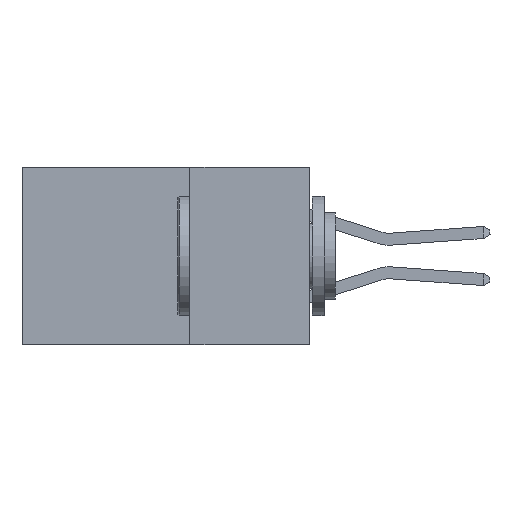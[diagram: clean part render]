
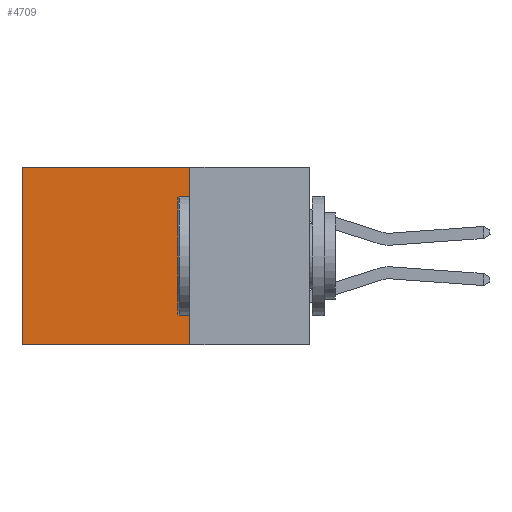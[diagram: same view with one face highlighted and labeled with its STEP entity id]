
A CAD part, left-side view. The second image highlights one B-rep face of the part: STEP entity #4709.
In plain terms, the highlighted planar face has unit normal (-1, 0, 0).
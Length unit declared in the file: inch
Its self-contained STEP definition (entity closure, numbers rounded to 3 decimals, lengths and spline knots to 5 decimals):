
#73 = CARTESIAN_POINT ( 'NONE',  ( 0.2615, 0.25, -0.37 ) ) ;
#1936 = ORIENTED_EDGE ( 'NONE', *, *, #3505, .F. ) ;
#3013 = ORIENTED_EDGE ( 'NONE', *, *, #3438, .F. ) ;
#3438 = EDGE_CURVE ( 'NONE', #7405, #14363, #18921, .T. ) ;
#3505 = EDGE_CURVE ( 'NONE', #14799, #7405, #18709, .T. ) ;
#4570 = VERTEX_POINT ( 'NONE', #19779 ) ;
#4709 = ADVANCED_FACE ( 'NONE', ( #9606 ), #11760, .F. ) ;
#5019 = ORIENTED_EDGE ( 'NONE', *, *, #10967, .T. ) ;
#6121 = LINE ( 'NONE', #10209, #7133 ) ;
#7133 = VECTOR ( 'NONE', #20650, 39.37008 ) ;
#7405 = VERTEX_POINT ( 'NONE', #14958 ) ;
#7559 = DIRECTION ( 'NONE',  ( 1., 0., 0. ) ) ;
#8209 = DIRECTION ( 'NONE',  ( 0., 0., -1. ) ) ;
#9606 = FACE_OUTER_BOUND ( 'NONE', #22116, .T. ) ;
#10209 = CARTESIAN_POINT ( 'NONE',  ( 0.2615, 0.6, -0.37 ) ) ;
#10636 = CARTESIAN_POINT ( 'NONE',  ( 0.2615, 0.25, 0. ) ) ;
#10967 = EDGE_CURVE ( 'NONE', #14799, #4570, #18759, .T. ) ;
#11760 = PLANE ( 'NONE',  #24007 ) ;
#14363 = VERTEX_POINT ( 'NONE', #17181 ) ;
#14706 = DIRECTION ( 'NONE',  ( 0., 1., 0. ) ) ;
#14799 = VERTEX_POINT ( 'NONE', #10636 ) ;
#14958 = CARTESIAN_POINT ( 'NONE',  ( 0.2615, 0.25, -0.37 ) ) ;
#14959 = DIRECTION ( 'NONE',  ( 0., 1., 0. ) ) ;
#16483 = EDGE_CURVE ( 'NONE', #4570, #14363, #6121, .T. ) ;
#17181 = CARTESIAN_POINT ( 'NONE',  ( 0.2615, 0.6, -0.37 ) ) ;
#17517 = VECTOR ( 'NONE', #14706, 39.37008 ) ;
#18709 = LINE ( 'NONE', #73, #21431 ) ;
#18759 = LINE ( 'NONE', #21352, #24596 ) ;
#18921 = LINE ( 'NONE', #22721, #17517 ) ;
#19779 = CARTESIAN_POINT ( 'NONE',  ( 0.2615, 0.6, 0. ) ) ;
#20042 = CARTESIAN_POINT ( 'NONE',  ( 0.2615, 0.25, -0.37 ) ) ;
#20650 = DIRECTION ( 'NONE',  ( 0., 0., -1. ) ) ;
#21352 = CARTESIAN_POINT ( 'NONE',  ( 0.2615, 0.25, 0. ) ) ;
#21431 = VECTOR ( 'NONE', #8209, 39.37008 ) ;
#22116 = EDGE_LOOP ( 'NONE', ( #24214, #3013, #1936, #5019 ) ) ;
#22721 = CARTESIAN_POINT ( 'NONE',  ( 0.2615, 0.25, -0.37 ) ) ;
#24007 = AXIS2_PLACEMENT_3D ( 'NONE', #20042, #7559, #24232 ) ;
#24214 = ORIENTED_EDGE ( 'NONE', *, *, #16483, .T. ) ;
#24232 = DIRECTION ( 'NONE',  ( 0., 0., -1. ) ) ;
#24596 = VECTOR ( 'NONE', #14959, 39.37008 ) ;
